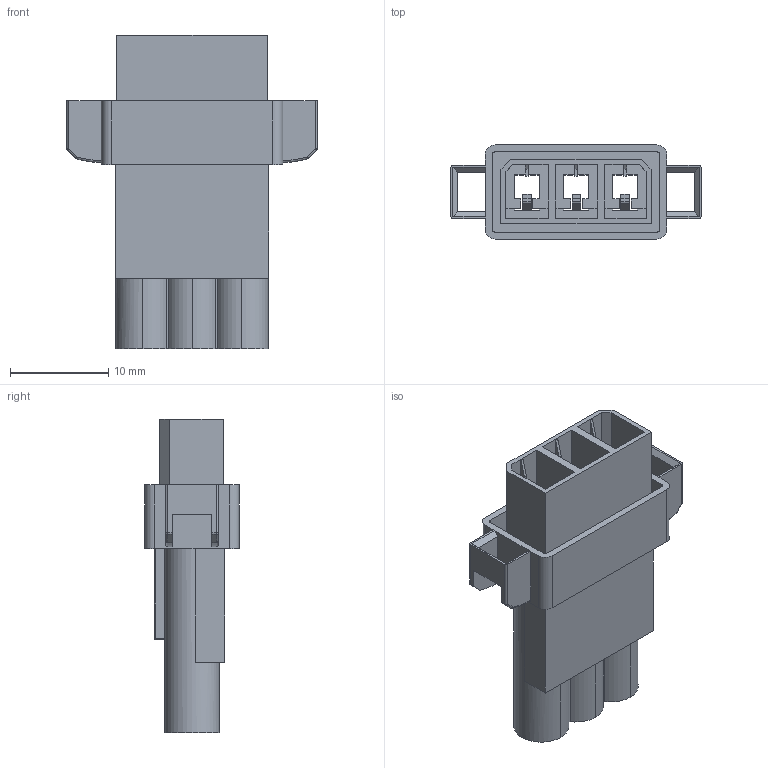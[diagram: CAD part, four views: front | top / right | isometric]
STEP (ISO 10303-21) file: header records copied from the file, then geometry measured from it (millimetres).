
FILE_DESCRIPTION (( 'STEP AP214' ), '1' );
FILE_NAME ('567-003-000-310.STEP', '2020-07-27T20:00:11', ( '' ), ( '' ), 'SwSTEP 2.0', 'SolidWorks 2020', '' );
FILE_SCHEMA (( 'AUTOMOTIVE_DESIGN' ));
Length unit declared in the file: millimetre
Products named in the file (1): 567-003-000-310
Bounding box: 25.5 x 9.6 x 32 mm (x, y, z)
Volume: 1579.9 mm3; surface area: 4240.1 mm2
Topology: 1 solids, 1 shells, 297 faces, 842 edges, 544 vertices
Faces by surface type: plane 216, cylinder 48, bspline 19, sphere 10, torus 4
Entity records: 10562 total; most frequent: CARTESIAN_POINT 2877, ORIENTED_EDGE 1672, DIRECTION 1486, EDGE_CURVE 836, VECTOR 644, LINE 644, VERTEX_POINT 544, AXIS2_PLACEMENT_3D 421
